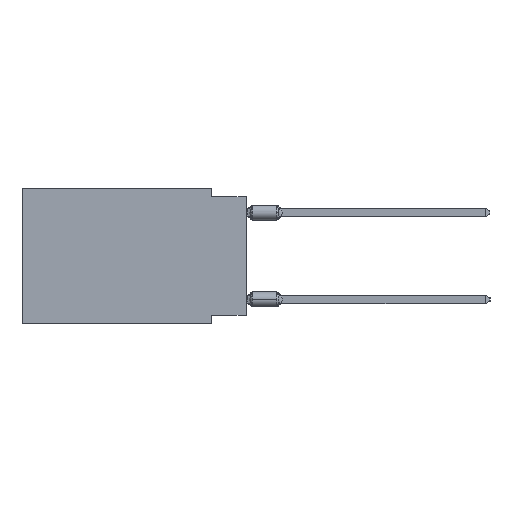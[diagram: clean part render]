
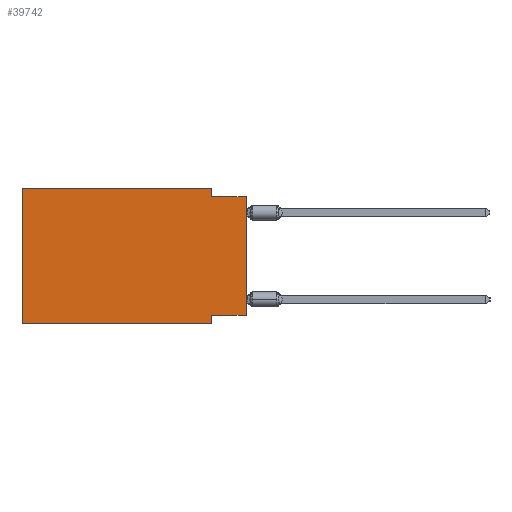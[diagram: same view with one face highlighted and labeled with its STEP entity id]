
A CAD part, left-side view. The second image highlights one B-rep face of the part: STEP entity #39742.
In plain terms, the highlighted planar face has unit normal (-1, 0, 0).
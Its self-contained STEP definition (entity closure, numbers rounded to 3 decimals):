
#2520 = DIRECTION ( 'NONE',  ( 0., 1., 0. ) ) ;
#3867 = CARTESIAN_POINT ( 'NONE',  ( 0., 0., -0.635 ) ) ;
#4297 = FACE_OUTER_BOUND ( 'NONE', #26207, .T. ) ;
#5551 = EDGE_CURVE ( 'NONE', #25458, #41575, #10236, .T. ) ;
#6102 = LINE ( 'NONE', #9249, #20810 ) ;
#8256 = VECTOR ( 'NONE', #49994, 1000. ) ;
#8559 = VECTOR ( 'NONE', #37609, 1000. ) ;
#9249 = CARTESIAN_POINT ( 'NONE',  ( 0., 2.54, 0. ) ) ;
#9370 = ORIENTED_EDGE ( 'NONE', *, *, #52864, .F. ) ;
#9806 = ORIENTED_EDGE ( 'NONE', *, *, #41026, .F. ) ;
#10236 = LINE ( 'NONE', #27628, #8559 ) ;
#10971 = ORIENTED_EDGE ( 'NONE', *, *, #42320, .F. ) ;
#11259 = CARTESIAN_POINT ( 'NONE',  ( 0., 2.54, -0.635 ) ) ;
#12039 = CARTESIAN_POINT ( 'NONE',  ( 0., 16.383, 0. ) ) ;
#13399 = DIRECTION ( 'NONE',  ( 0., 0., -1. ) ) ;
#13596 = ORIENTED_EDGE ( 'NONE', *, *, #53783, .F. ) ;
#13801 = EDGE_CURVE ( 'NONE', #54451, #45616, #16982, .T. ) ;
#14492 = CARTESIAN_POINT ( 'NONE',  ( 0., 16.383, -9.906 ) ) ;
#14876 = CARTESIAN_POINT ( 'NONE',  ( 0., 16.383, 0. ) ) ;
#15160 = LINE ( 'NONE', #14876, #8256 ) ;
#16028 = VERTEX_POINT ( 'NONE', #11259 ) ;
#16135 = DIRECTION ( 'NONE',  ( 0., 0., 1. ) ) ;
#16982 = LINE ( 'NONE', #21275, #46217 ) ;
#19451 = VECTOR ( 'NONE', #51819, 1000. ) ;
#19767 = VECTOR ( 'NONE', #44881, 1000. ) ;
#19860 = ORIENTED_EDGE ( 'NONE', *, *, #35080, .F. ) ;
#20810 = VECTOR ( 'NONE', #39786, 1000. ) ;
#21275 = CARTESIAN_POINT ( 'NONE',  ( 0., 0., 0. ) ) ;
#21713 = PLANE ( 'NONE',  #31525 ) ;
#22224 = CARTESIAN_POINT ( 'NONE',  ( 0., 16.383, 0. ) ) ;
#24173 = CARTESIAN_POINT ( 'NONE',  ( 0., 0., -0.635 ) ) ;
#25458 = VERTEX_POINT ( 'NONE', #14492 ) ;
#26207 = EDGE_LOOP ( 'NONE', ( #51484, #19860, #13596, #10971, #40312, #56047, #9806, #9370 ) ) ;
#26573 = EDGE_CURVE ( 'NONE', #25458, #33931, #52482, .T. ) ;
#26673 = VERTEX_POINT ( 'NONE', #55561 ) ;
#27628 = CARTESIAN_POINT ( 'NONE',  ( 0., 16.383, -9.906 ) ) ;
#28793 = LINE ( 'NONE', #50515, #19767 ) ;
#29587 = CARTESIAN_POINT ( 'NONE',  ( 0., 2.54, -9.906 ) ) ;
#29722 = VECTOR ( 'NONE', #52761, 1000. ) ;
#31525 = AXIS2_PLACEMENT_3D ( 'NONE', #39390, #39115, #13399 ) ;
#33931 = VERTEX_POINT ( 'NONE', #12039 ) ;
#34120 = LINE ( 'NONE', #3867, #19451 ) ;
#35080 = EDGE_CURVE ( 'NONE', #16028, #45616, #34120, .T. ) ;
#36853 = VERTEX_POINT ( 'NONE', #42906 ) ;
#37609 = DIRECTION ( 'NONE',  ( 0., -1., 0. ) ) ;
#39115 = DIRECTION ( 'NONE',  ( 1., 0., 0. ) ) ;
#39390 = CARTESIAN_POINT ( 'NONE',  ( 0., 16.383, 0. ) ) ;
#39742 = ADVANCED_FACE ( 'NONE', ( #4297 ), #21713, .F. ) ;
#39756 = VECTOR ( 'NONE', #2520, 1000. ) ;
#39786 = DIRECTION ( 'NONE',  ( 0., 0., -1. ) ) ;
#40312 = ORIENTED_EDGE ( 'NONE', *, *, #26573, .F. ) ;
#41026 = EDGE_CURVE ( 'NONE', #36853, #41575, #28793, .T. ) ;
#41575 = VERTEX_POINT ( 'NONE', #29587 ) ;
#42320 = EDGE_CURVE ( 'NONE', #33931, #26673, #15160, .T. ) ;
#42906 = CARTESIAN_POINT ( 'NONE',  ( 0., 2.54, -9.271 ) ) ;
#44460 = CARTESIAN_POINT ( 'NONE',  ( 0., 0., -9.271 ) ) ;
#44881 = DIRECTION ( 'NONE',  ( 0., 0., -1. ) ) ;
#45616 = VERTEX_POINT ( 'NONE', #24173 ) ;
#46217 = VECTOR ( 'NONE', #16135, 1000. ) ;
#48773 = LINE ( 'NONE', #51324, #39756 ) ;
#49994 = DIRECTION ( 'NONE',  ( 0., -1., 0. ) ) ;
#50515 = CARTESIAN_POINT ( 'NONE',  ( 0., 2.54, -9.906 ) ) ;
#51324 = CARTESIAN_POINT ( 'NONE',  ( 0., 0., -9.271 ) ) ;
#51484 = ORIENTED_EDGE ( 'NONE', *, *, #13801, .T. ) ;
#51819 = DIRECTION ( 'NONE',  ( 0., -1., 0. ) ) ;
#52482 = LINE ( 'NONE', #22224, #29722 ) ;
#52761 = DIRECTION ( 'NONE',  ( 0., 0., 1. ) ) ;
#52864 = EDGE_CURVE ( 'NONE', #54451, #36853, #48773, .T. ) ;
#53783 = EDGE_CURVE ( 'NONE', #26673, #16028, #6102, .T. ) ;
#54451 = VERTEX_POINT ( 'NONE', #44460 ) ;
#55561 = CARTESIAN_POINT ( 'NONE',  ( 0., 2.54, 0. ) ) ;
#56047 = ORIENTED_EDGE ( 'NONE', *, *, #5551, .T. ) ;
